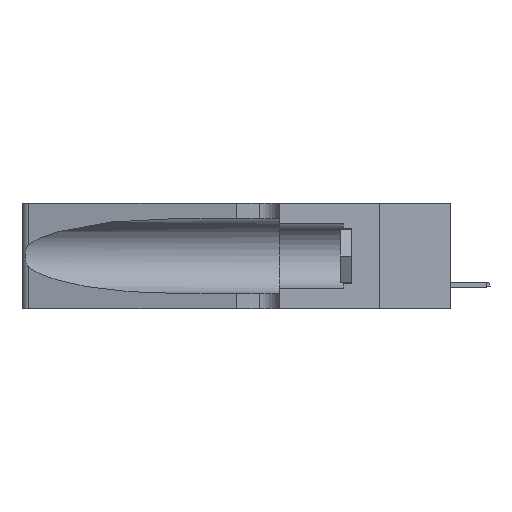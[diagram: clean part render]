
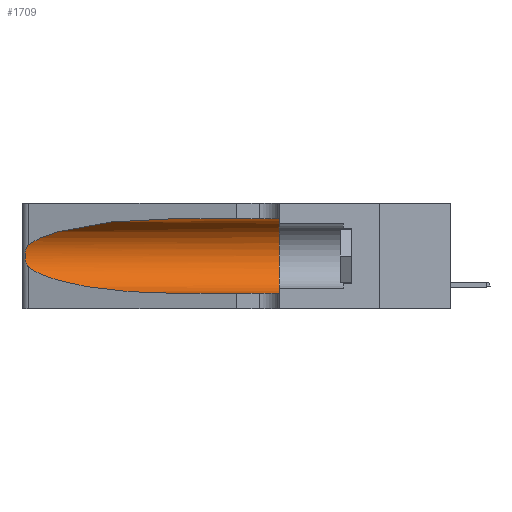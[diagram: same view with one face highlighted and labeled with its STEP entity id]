
A CAD part, left-side view. The second image highlights one B-rep face of the part: STEP entity #1709.
In plain terms, the highlighted cylindrical face has radius 3.308 mm (diameter 6.617 mm), a partial arc.
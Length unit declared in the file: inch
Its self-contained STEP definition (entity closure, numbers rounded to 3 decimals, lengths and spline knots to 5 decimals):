
#118 = EDGE_CURVE ( 'NONE', #574, #5414, #21574, .T. ) ;
#574 = VERTEX_POINT ( 'NONE', #10753 ) ;
#1266 = CARTESIAN_POINT ( 'NONE',  ( 0.1305, 0.35, 0.05475 ) ) ;
#1306 = DIRECTION ( 'NONE',  ( 0., 1., 0. ) ) ;
#1365 = EDGE_CURVE ( 'NONE', #6135, #574, #12719, .T. ) ;
#1598 = DIRECTION ( 'NONE',  ( 0., -1., 0. ) ) ;
#1709 = ADVANCED_FACE ( 'NONE', ( #15855 ), #14115, .F. ) ;
#1881 = CARTESIAN_POINT ( 'NONE',  ( 0.2373, 1.15595, 0.08982 ) ) ;
#1926 = CARTESIAN_POINT ( 'NONE',  ( 0.1305, 0.72297, 0.31525 ) ) ;
#2089 = ORIENTED_EDGE ( 'NONE', *, *, #18253, .F. ) ;
#2478 = ORIENTED_EDGE ( 'NONE', *, *, #21514, .T. ) ;
#2961 = CARTESIAN_POINT ( 'NONE',  ( 0.25487, 1.22718, 0.22369 ) ) ;
#3086 =( BOUNDED_CURVE ( )  B_SPLINE_CURVE ( 3, ( #18858, #12028, #6750, #21041 ),
 .UNSPECIFIED., .F., .T. ) 
 B_SPLINE_CURVE_WITH_KNOTS ( ( 4, 4 ),
 ( 1.5708, 2.84003 ),
 .UNSPECIFIED. ) 
 CURVE ( )  GEOMETRIC_REPRESENTATION_ITEM ( )  RATIONAL_B_SPLINE_CURVE ( ( 1., 0.87, 0.87, 1. ) ) 
 REPRESENTATION_ITEM ( '' )  );
#3229 = VERTEX_POINT ( 'NONE', #14543 ) ;
#3298 = CARTESIAN_POINT ( 'NONE',  ( 0.25639, 1.23186, 0.15144 ) ) ;
#3338 = EDGE_CURVE ( 'NONE', #5765, #6135, #3507, .T. ) ;
#3419 = ORIENTED_EDGE ( 'NONE', *, *, #1365, .T. ) ;
#3507 = B_SPLINE_CURVE_WITH_KNOTS ( 'NONE', 3,
 ( #2961, #9956, #16965, #4698, #18841, #11911, #8572, #8343, #22294, #20576, #10068, #3298, #17078, #22403 ),
 .UNSPECIFIED., .F., .F.,
 ( 4, 2, 2, 2, 2, 2, 4 ),
 ( 0., 0.00027, 0.00053, 0.00107, 0.0016, 0.00187, 0.00214 ),
 .UNSPECIFIED. ) ;
#4698 = CARTESIAN_POINT ( 'NONE',  ( 0.25787, 1.23484, 0.2124 ) ) ;
#5414 = VERTEX_POINT ( 'NONE', #1266 ) ;
#5765 = VERTEX_POINT ( 'NONE', #8457 ) ;
#5997 = DIRECTION ( 'NONE',  ( 0., -1., 0. ) ) ;
#6135 = VERTEX_POINT ( 'NONE', #22002 ) ;
#6750 = CARTESIAN_POINT ( 'NONE',  ( 0.2373, 1.15595, 0.28018 ) ) ;
#8343 = CARTESIAN_POINT ( 'NONE',  ( 0.26075, 1.23896, 0.178 ) ) ;
#8457 = CARTESIAN_POINT ( 'NONE',  ( 0.25487, 1.22718, 0.22369 ) ) ;
#8572 = CARTESIAN_POINT ( 'NONE',  ( 0.26075, 1.23896, 0.19203 ) ) ;
#8775 = CARTESIAN_POINT ( 'NONE',  ( 0.1305, 0.72297, 0.05475 ) ) ;
#9585 = CARTESIAN_POINT ( 'NONE',  ( 0.1305, 1.61858, 0.05475 ) ) ;
#9956 = CARTESIAN_POINT ( 'NONE',  ( 0.25555, 1.22994, 0.2215 ) ) ;
#10037 = CARTESIAN_POINT ( 'NONE',  ( 0.1305, 0.35, 0.185 ) ) ;
#10068 = CARTESIAN_POINT ( 'NONE',  ( 0.25789, 1.23486, 0.15765 ) ) ;
#10141 = ORIENTED_EDGE ( 'NONE', *, *, #118, .T. ) ;
#10345 = DIRECTION ( 'NONE',  ( 0., -1., 0. ) ) ;
#10753 = CARTESIAN_POINT ( 'NONE',  ( 0.1305, 0.72297, 0.05475 ) ) ;
#11710 = VECTOR ( 'NONE', #5997, 39.37008 ) ;
#11911 = CARTESIAN_POINT ( 'NONE',  ( 0.26018, 1.23835, 0.19895 ) ) ;
#12028 = CARTESIAN_POINT ( 'NONE',  ( 0.18966, 0.96281, 0.31525 ) ) ;
#12719 =( BOUNDED_CURVE ( )  B_SPLINE_CURVE ( 3, ( #22483, #1881, #19165, #8775 ),
 .UNSPECIFIED., .F., .T. ) 
 B_SPLINE_CURVE_WITH_KNOTS ( ( 4, 4 ),
 ( 3.44316, 4.71239 ),
 .UNSPECIFIED. ) 
 CURVE ( )  GEOMETRIC_REPRESENTATION_ITEM ( )  RATIONAL_B_SPLINE_CURVE ( ( 1., 0.87, 0.87, 1. ) ) 
 REPRESENTATION_ITEM ( '' )  );
#13682 = VECTOR ( 'NONE', #1598, 39.37008 ) ;
#14090 = CARTESIAN_POINT ( 'NONE',  ( 0.1305, 1.61858, 0.31525 ) ) ;
#14115 = CYLINDRICAL_SURFACE ( 'NONE', #14290, 0.13025 ) ;
#14290 = AXIS2_PLACEMENT_3D ( 'NONE', #15393, #10345, #19027 ) ;
#14543 = CARTESIAN_POINT ( 'NONE',  ( 0.1305, 0.35, 0.31525 ) ) ;
#14689 = ORIENTED_EDGE ( 'NONE', *, *, #3338, .T. ) ;
#15308 = DIRECTION ( 'NONE',  ( 0., 0., 1. ) ) ;
#15393 = CARTESIAN_POINT ( 'NONE',  ( 0.1305, 1.61858, 0.185 ) ) ;
#15700 = LINE ( 'NONE', #14090, #13682 ) ;
#15855 = FACE_OUTER_BOUND ( 'NONE', #20856, .T. ) ;
#16491 = EDGE_CURVE ( 'NONE', #3229, #5414, #20683, .T. ) ;
#16965 = CARTESIAN_POINT ( 'NONE',  ( 0.25639, 1.23184, 0.21858 ) ) ;
#17054 = VERTEX_POINT ( 'NONE', #1926 ) ;
#17078 = CARTESIAN_POINT ( 'NONE',  ( 0.25555, 1.22993, 0.14849 ) ) ;
#18253 = EDGE_CURVE ( 'NONE', #17054, #3229, #15700, .T. ) ;
#18841 = CARTESIAN_POINT ( 'NONE',  ( 0.25854, 1.2359, 0.20912 ) ) ;
#18858 = CARTESIAN_POINT ( 'NONE',  ( 0.1305, 0.72297, 0.31525 ) ) ;
#19027 = DIRECTION ( 'NONE',  ( 0., 0., -1. ) ) ;
#19165 = CARTESIAN_POINT ( 'NONE',  ( 0.18966, 0.96281, 0.05475 ) ) ;
#19520 = ORIENTED_EDGE ( 'NONE', *, *, #16491, .F. ) ;
#20576 = CARTESIAN_POINT ( 'NONE',  ( 0.25856, 1.23593, 0.16098 ) ) ;
#20683 = CIRCLE ( 'NONE', #21800, 0.13025 ) ;
#20856 = EDGE_LOOP ( 'NONE', ( #2478, #14689, #3419, #10141, #19520, #2089 ) ) ;
#21041 = CARTESIAN_POINT ( 'NONE',  ( 0.25487, 1.22718, 0.22369 ) ) ;
#21514 = EDGE_CURVE ( 'NONE', #17054, #5765, #3086, .T. ) ;
#21574 = LINE ( 'NONE', #9585, #11710 ) ;
#21800 = AXIS2_PLACEMENT_3D ( 'NONE', #10037, #1306, #15308 ) ;
#22002 = CARTESIAN_POINT ( 'NONE',  ( 0.25487, 1.22718, 0.14631 ) ) ;
#22294 = CARTESIAN_POINT ( 'NONE',  ( 0.26017, 1.23833, 0.17102 ) ) ;
#22403 = CARTESIAN_POINT ( 'NONE',  ( 0.25487, 1.22718, 0.14631 ) ) ;
#22483 = CARTESIAN_POINT ( 'NONE',  ( 0.25487, 1.22718, 0.14631 ) ) ;
